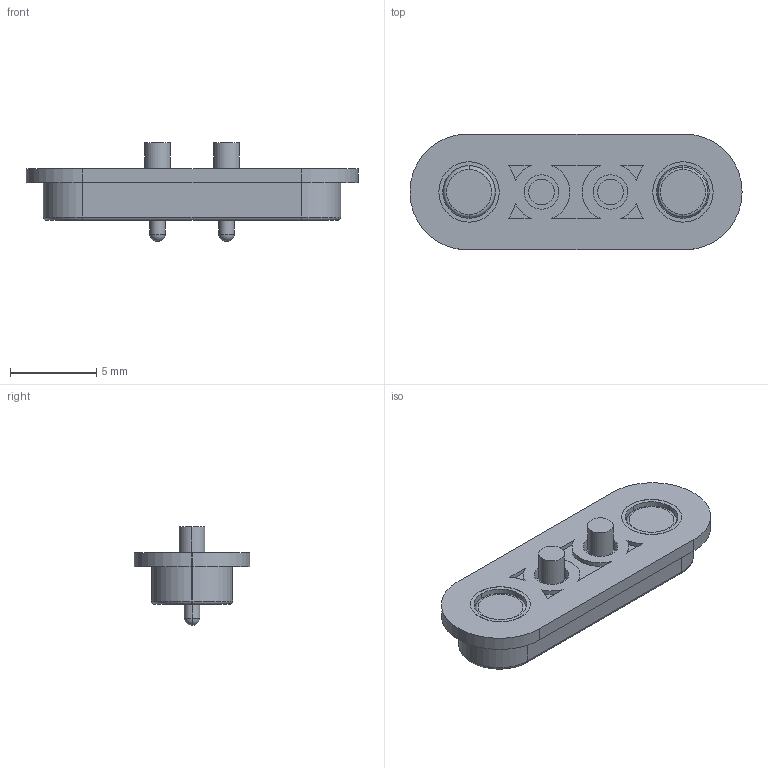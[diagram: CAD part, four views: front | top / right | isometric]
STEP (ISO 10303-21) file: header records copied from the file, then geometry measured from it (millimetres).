
FILE_DESCRIPTION (( 'STEP AP214' ), '1' );
FILE_NAME ('685L0222211110E.STEP', '2023-04-13T19:52:26', ( '' ), ( '' ), 'SwSTEP 2.0', 'SolidWorks 2020', '' );
FILE_SCHEMA (( 'AUTOMOTIVE_DESIGN' ));
Length unit declared in the file: millimetre
Products named in the file (1): 685L0222211110E
Bounding box: 19.25 x 6.7 x 5.7 mm (x, y, z)
Volume: 260.4 mm3; surface area: 464.8 mm2
Topology: 5 solids, 5 shells, 133 faces, 289 edges, 184 vertices
Faces by surface type: cylinder 55, plane 54, torus 18, cone 4, bspline 2
Entity records: 5266 total; most frequent: CARTESIAN_POINT 737, DIRECTION 695, ORIENTED_EDGE 578, EDGE_CURVE 289, AXIS2_PLACEMENT_3D 278, VERTEX_POINT 184, EDGE_LOOP 151, CIRCLE 146
